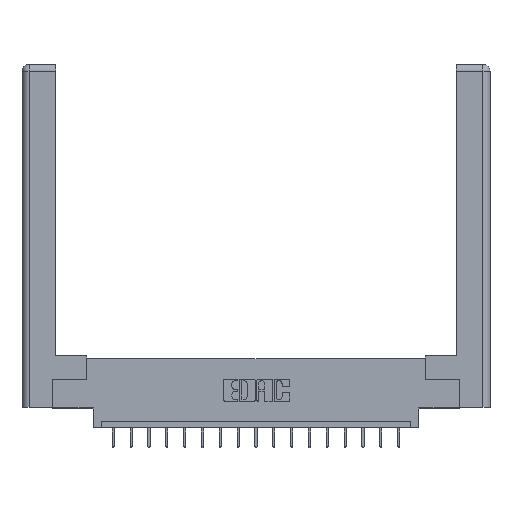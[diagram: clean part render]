
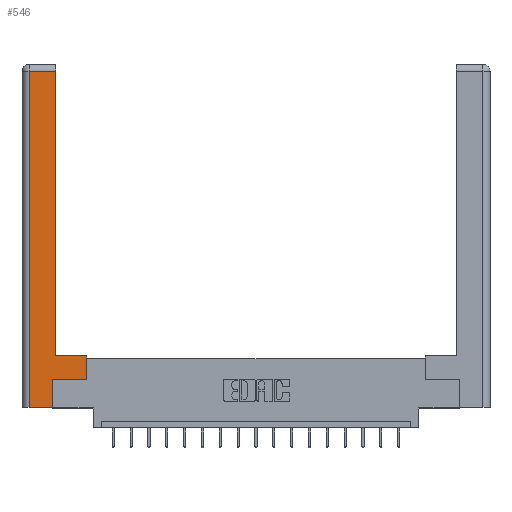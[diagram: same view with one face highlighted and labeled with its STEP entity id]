
A CAD part, top view. The second image highlights one B-rep face of the part: STEP entity #546.
In plain terms, the highlighted planar face has unit normal (0, 0, 1).
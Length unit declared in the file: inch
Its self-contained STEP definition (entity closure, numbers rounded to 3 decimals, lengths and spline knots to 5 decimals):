
#473 = DIRECTION ( 'NONE',  ( -1., 0., 0. ) ) ;
#546 = ADVANCED_FACE ( 'NONE', ( #900 ), #12407, .F. ) ;
#683 = DIRECTION ( 'NONE',  ( 1., 0., 0. ) ) ;
#900 = FACE_OUTER_BOUND ( 'NONE', #15886, .T. ) ;
#962 = EDGE_CURVE ( 'NONE', #14452, #2081, #4426, .T. ) ;
#1013 = ORIENTED_EDGE ( 'NONE', *, *, #9475, .T. ) ;
#1083 = LINE ( 'NONE', #10728, #6109 ) ;
#1636 = CARTESIAN_POINT ( 'NONE',  ( 0.0615, 0., 0. ) ) ;
#1805 = DIRECTION ( 'NONE',  ( 0., 1., 0. ) ) ;
#2081 = VERTEX_POINT ( 'NONE', #5120 ) ;
#2303 = EDGE_CURVE ( 'NONE', #15968, #5159, #10919, .T. ) ;
#2415 = DIRECTION ( 'NONE',  ( 0., 0., -1. ) ) ;
#2661 = CARTESIAN_POINT ( 'NONE',  ( 0.295, 0.45, 0. ) ) ;
#2693 = LINE ( 'NONE', #3182, #3222 ) ;
#2724 = VECTOR ( 'NONE', #683, 39.37008 ) ;
#2792 = DIRECTION ( 'NONE',  ( 0., 1., 0. ) ) ;
#2846 = EDGE_CURVE ( 'NONE', #6125, #13216, #12675, .T. ) ;
#3031 = CARTESIAN_POINT ( 'NONE',  ( 0.265, 0.245, 0. ) ) ;
#3182 = CARTESIAN_POINT ( 'NONE',  ( 0.295, 3., 0. ) ) ;
#3222 = VECTOR ( 'NONE', #12015, 39.37008 ) ;
#3773 = DIRECTION ( 'NONE',  ( 0., -1., 0. ) ) ;
#3866 = LINE ( 'NONE', #4792, #7283 ) ;
#4313 = EDGE_CURVE ( 'NONE', #5159, #14452, #2693, .T. ) ;
#4426 = LINE ( 'NONE', #8974, #8022 ) ;
#4792 = CARTESIAN_POINT ( 'NONE',  ( 0.565, 0.45, 0. ) ) ;
#5120 = CARTESIAN_POINT ( 'NONE',  ( 0.0615, 2.94, 0. ) ) ;
#5159 = VERTEX_POINT ( 'NONE', #2661 ) ;
#5215 = VERTEX_POINT ( 'NONE', #17063 ) ;
#5286 = ORIENTED_EDGE ( 'NONE', *, *, #962, .T. ) ;
#5849 = CARTESIAN_POINT ( 'NONE',  ( 0.265, 0., 0. ) ) ;
#5934 = VECTOR ( 'NONE', #473, 39.37008 ) ;
#6109 = VECTOR ( 'NONE', #3773, 39.37008 ) ;
#6125 = VERTEX_POINT ( 'NONE', #1636 ) ;
#6213 = LINE ( 'NONE', #7487, #13447 ) ;
#7283 = VECTOR ( 'NONE', #1805, 39.37008 ) ;
#7487 = CARTESIAN_POINT ( 'NONE',  ( 0.565, 0.245, 0. ) ) ;
#8022 = VECTOR ( 'NONE', #11547, 39.37008 ) ;
#8701 = CARTESIAN_POINT ( 'NONE',  ( 0.565, 0.45, 0. ) ) ;
#8974 = CARTESIAN_POINT ( 'NONE',  ( 0.0615, 2.94, 0. ) ) ;
#9316 = CARTESIAN_POINT ( 'NONE',  ( 0.265, 0., 0. ) ) ;
#9475 = EDGE_CURVE ( 'NONE', #13216, #11057, #12203, .T. ) ;
#9746 = VECTOR ( 'NONE', #2792, 39.37008 ) ;
#10691 = ORIENTED_EDGE ( 'NONE', *, *, #18657, .T. ) ;
#10728 = CARTESIAN_POINT ( 'NONE',  ( 0.0615, 0., 0. ) ) ;
#10875 = CARTESIAN_POINT ( 'NONE',  ( 0.295, 0.45, 0. ) ) ;
#10919 = LINE ( 'NONE', #10875, #5934 ) ;
#11057 = VERTEX_POINT ( 'NONE', #3031 ) ;
#11304 = ORIENTED_EDGE ( 'NONE', *, *, #4313, .T. ) ;
#11366 = ORIENTED_EDGE ( 'NONE', *, *, #12327, .T. ) ;
#11461 = CARTESIAN_POINT ( 'NONE',  ( 0.295, 2.94, 0. ) ) ;
#11547 = DIRECTION ( 'NONE',  ( -1., 0., 0. ) ) ;
#12015 = DIRECTION ( 'NONE',  ( 0., 1., 0. ) ) ;
#12203 = LINE ( 'NONE', #14243, #9746 ) ;
#12327 = EDGE_CURVE ( 'NONE', #11057, #5215, #6213, .T. ) ;
#12407 = PLANE ( 'NONE',  #18258 ) ;
#12527 = DIRECTION ( 'NONE',  ( -1., 0., 0. ) ) ;
#12675 = LINE ( 'NONE', #9316, #2724 ) ;
#13109 = ORIENTED_EDGE ( 'NONE', *, *, #2303, .T. ) ;
#13216 = VERTEX_POINT ( 'NONE', #5849 ) ;
#13447 = VECTOR ( 'NONE', #17469, 39.37008 ) ;
#14243 = CARTESIAN_POINT ( 'NONE',  ( 0.265, 0.245, 0. ) ) ;
#14430 = ORIENTED_EDGE ( 'NONE', *, *, #2846, .T. ) ;
#14452 = VERTEX_POINT ( 'NONE', #11461 ) ;
#15886 = EDGE_LOOP ( 'NONE', ( #11304, #5286, #10691, #14430, #1013, #11366, #16902, #13109 ) ) ;
#15968 = VERTEX_POINT ( 'NONE', #8701 ) ;
#16813 = CARTESIAN_POINT ( 'NONE',  ( 0., 0., 0. ) ) ;
#16902 = ORIENTED_EDGE ( 'NONE', *, *, #17357, .T. ) ;
#17063 = CARTESIAN_POINT ( 'NONE',  ( 0.565, 0.245, 0. ) ) ;
#17357 = EDGE_CURVE ( 'NONE', #5215, #15968, #3866, .T. ) ;
#17469 = DIRECTION ( 'NONE',  ( 1., 0., 0. ) ) ;
#18258 = AXIS2_PLACEMENT_3D ( 'NONE', #16813, #2415, #12527 ) ;
#18657 = EDGE_CURVE ( 'NONE', #2081, #6125, #1083, .T. ) ;
